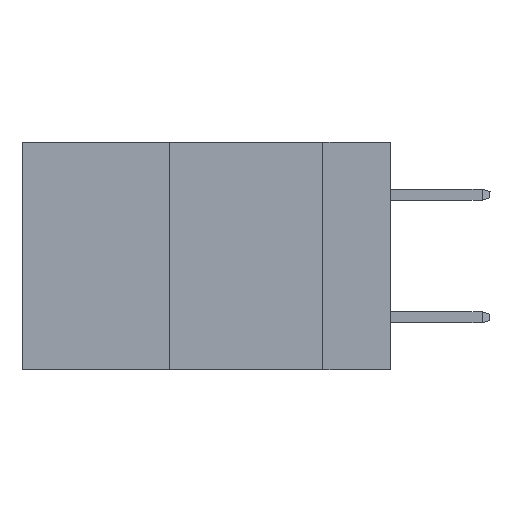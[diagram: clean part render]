
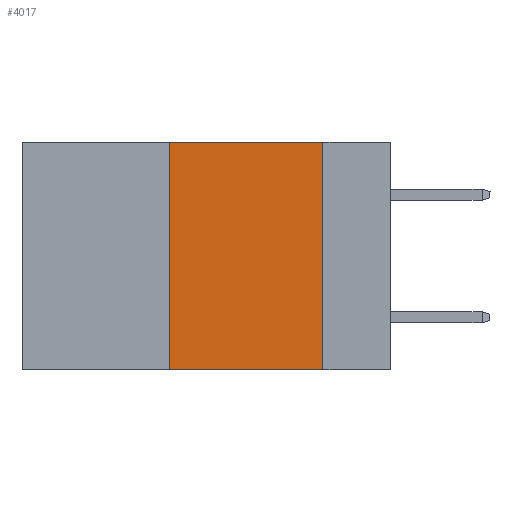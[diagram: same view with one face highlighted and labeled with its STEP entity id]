
A CAD part, left-side view. The second image highlights one B-rep face of the part: STEP entity #4017.
In plain terms, the highlighted planar face has unit normal (-1, 0, 0).
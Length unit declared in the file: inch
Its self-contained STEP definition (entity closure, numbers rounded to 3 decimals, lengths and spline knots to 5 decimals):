
#106 = VERTEX_POINT ( 'NONE', #855 ) ;
#335 = PLANE ( 'NONE',  #1508 ) ;
#406 = CARTESIAN_POINT ( 'NONE',  ( 0., 0.11, 0. ) ) ;
#855 = CARTESIAN_POINT ( 'NONE',  ( 0., 0.11, -0.37 ) ) ;
#1195 = CARTESIAN_POINT ( 'NONE',  ( 0., 0.11, 0. ) ) ;
#1290 = VERTEX_POINT ( 'NONE', #7478 ) ;
#1408 = CARTESIAN_POINT ( 'NONE',  ( 0., 0.6, -0.37 ) ) ;
#1508 = AXIS2_PLACEMENT_3D ( 'NONE', #10737, #10590, #6357 ) ;
#1582 = DIRECTION ( 'NONE',  ( 0., -1., 0. ) ) ;
#1623 = ORIENTED_EDGE ( 'NONE', *, *, #2288, .F. ) ;
#1840 = VECTOR ( 'NONE', #10773, 39.37008 ) ;
#1974 = LINE ( 'NONE', #4919, #1840 ) ;
#2288 = EDGE_CURVE ( 'NONE', #1290, #6406, #3123, .T. ) ;
#2532 = VECTOR ( 'NONE', #10000, 39.37008 ) ;
#3123 = LINE ( 'NONE', #11067, #6768 ) ;
#3447 = ORIENTED_EDGE ( 'NONE', *, *, #4734, .T. ) ;
#3889 = CARTESIAN_POINT ( 'NONE',  ( 0., 0.36, -0.37 ) ) ;
#4017 = ADVANCED_FACE ( 'NONE', ( #7649 ), #335, .F. ) ;
#4720 = VERTEX_POINT ( 'NONE', #3889 ) ;
#4734 = EDGE_CURVE ( 'NONE', #4720, #106, #7640, .T. ) ;
#4919 = CARTESIAN_POINT ( 'NONE',  ( 0., 0.36, 0. ) ) ;
#6357 = DIRECTION ( 'NONE',  ( 0., 0., -1. ) ) ;
#6406 = VERTEX_POINT ( 'NONE', #1195 ) ;
#6768 = VECTOR ( 'NONE', #1582, 39.37008 ) ;
#6881 = ORIENTED_EDGE ( 'NONE', *, *, #8205, .F. ) ;
#6945 = LINE ( 'NONE', #406, #7351 ) ;
#7351 = VECTOR ( 'NONE', #9759, 39.37008 ) ;
#7478 = CARTESIAN_POINT ( 'NONE',  ( 0., 0.36, 0. ) ) ;
#7640 = LINE ( 'NONE', #1408, #2532 ) ;
#7649 = FACE_OUTER_BOUND ( 'NONE', #9024, .T. ) ;
#8057 = EDGE_CURVE ( 'NONE', #6406, #106, #6945, .T. ) ;
#8205 = EDGE_CURVE ( 'NONE', #4720, #1290, #1974, .T. ) ;
#9024 = EDGE_LOOP ( 'NONE', ( #10113, #1623, #6881, #3447 ) ) ;
#9759 = DIRECTION ( 'NONE',  ( 0., 0., -1. ) ) ;
#10000 = DIRECTION ( 'NONE',  ( 0., -1., 0. ) ) ;
#10113 = ORIENTED_EDGE ( 'NONE', *, *, #8057, .F. ) ;
#10590 = DIRECTION ( 'NONE',  ( 1., 0., 0. ) ) ;
#10737 = CARTESIAN_POINT ( 'NONE',  ( 0., 0.6, 0. ) ) ;
#10773 = DIRECTION ( 'NONE',  ( 0., 0., 1. ) ) ;
#11067 = CARTESIAN_POINT ( 'NONE',  ( 0., 0.6, 0. ) ) ;
